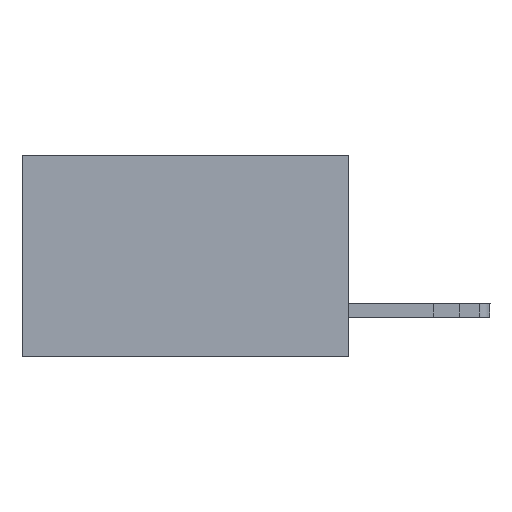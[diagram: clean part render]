
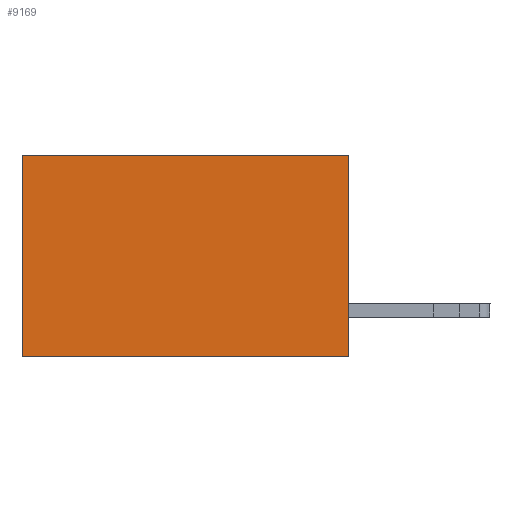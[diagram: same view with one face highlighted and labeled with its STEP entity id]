
A CAD part, left-side view. The second image highlights one B-rep face of the part: STEP entity #9169.
In plain terms, the highlighted planar face has unit normal (-1, 0, 0).
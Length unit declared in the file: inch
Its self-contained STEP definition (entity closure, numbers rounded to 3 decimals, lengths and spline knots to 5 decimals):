
#94 = DIRECTION ( 'NONE',  ( 1., 0., 0. ) ) ;
#1065 = VECTOR ( 'NONE', #12275, 39.37008 ) ;
#1365 = EDGE_CURVE ( 'NONE', #2936, #3119, #6649, .T. ) ;
#1413 = CARTESIAN_POINT ( 'NONE',  ( 0.2615, 0.6, 0. ) ) ;
#1744 = CARTESIAN_POINT ( 'NONE',  ( 0.2615, 0., -0.37 ) ) ;
#1933 = DIRECTION ( 'NONE',  ( 0., 0., -1. ) ) ;
#2057 = EDGE_CURVE ( 'NONE', #3119, #15382, #4729, .T. ) ;
#2936 = VERTEX_POINT ( 'NONE', #8236 ) ;
#3119 = VERTEX_POINT ( 'NONE', #1413 ) ;
#3432 = LINE ( 'NONE', #1744, #16465 ) ;
#3439 = ORIENTED_EDGE ( 'NONE', *, *, #2057, .T. ) ;
#3473 = CARTESIAN_POINT ( 'NONE',  ( 0.2615, 0., -0.37 ) ) ;
#3532 = EDGE_CURVE ( 'NONE', #13160, #15382, #3432, .T. ) ;
#3616 = ORIENTED_EDGE ( 'NONE', *, *, #3532, .F. ) ;
#4071 = ORIENTED_EDGE ( 'NONE', *, *, #7940, .F. ) ;
#4111 = ORIENTED_EDGE ( 'NONE', *, *, #1365, .T. ) ;
#4729 = LINE ( 'NONE', #14789, #1065 ) ;
#4789 = LINE ( 'NONE', #9730, #14440 ) ;
#5876 = DIRECTION ( 'NONE',  ( 0., 1., 0. ) ) ;
#6649 = LINE ( 'NONE', #14156, #12867 ) ;
#6928 = PLANE ( 'NONE',  #12688 ) ;
#7940 = EDGE_CURVE ( 'NONE', #2936, #13160, #4789, .T. ) ;
#8236 = CARTESIAN_POINT ( 'NONE',  ( 0.2615, 0., 0. ) ) ;
#8574 = DIRECTION ( 'NONE',  ( 0., 1., 0. ) ) ;
#9169 = ADVANCED_FACE ( 'NONE', ( #9192 ), #6928, .F. ) ;
#9192 = FACE_OUTER_BOUND ( 'NONE', #11169, .T. ) ;
#9385 = DIRECTION ( 'NONE',  ( 0., 0., -1. ) ) ;
#9730 = CARTESIAN_POINT ( 'NONE',  ( 0.2615, 0., -0.37 ) ) ;
#11169 = EDGE_LOOP ( 'NONE', ( #3439, #3616, #4071, #4111 ) ) ;
#11207 = CARTESIAN_POINT ( 'NONE',  ( 0.2615, 0.6, -0.37 ) ) ;
#12275 = DIRECTION ( 'NONE',  ( 0., 0., -1. ) ) ;
#12688 = AXIS2_PLACEMENT_3D ( 'NONE', #15588, #94, #9385 ) ;
#12867 = VECTOR ( 'NONE', #8574, 39.37008 ) ;
#13160 = VERTEX_POINT ( 'NONE', #3473 ) ;
#14156 = CARTESIAN_POINT ( 'NONE',  ( 0.2615, 0., 0. ) ) ;
#14440 = VECTOR ( 'NONE', #1933, 39.37008 ) ;
#14789 = CARTESIAN_POINT ( 'NONE',  ( 0.2615, 0.6, -0.37 ) ) ;
#15382 = VERTEX_POINT ( 'NONE', #11207 ) ;
#15588 = CARTESIAN_POINT ( 'NONE',  ( 0.2615, 0., -0.37 ) ) ;
#16465 = VECTOR ( 'NONE', #5876, 39.37008 ) ;
